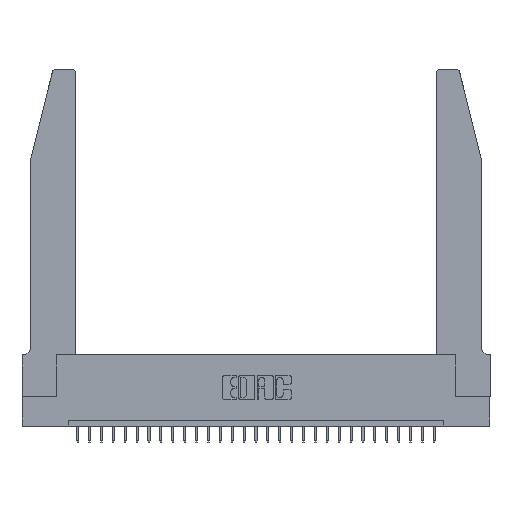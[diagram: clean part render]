
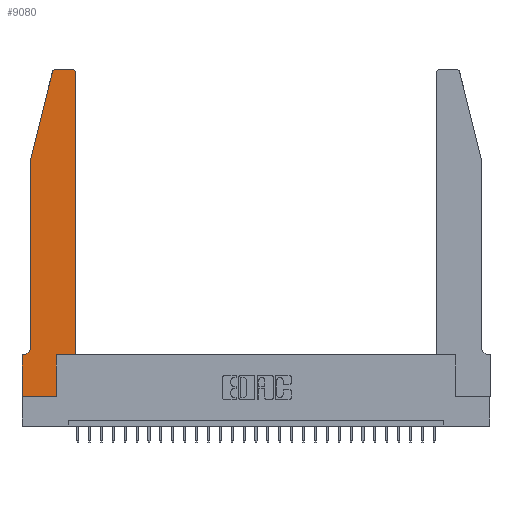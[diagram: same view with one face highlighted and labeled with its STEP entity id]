
A CAD part, top view. The second image highlights one B-rep face of the part: STEP entity #9080.
In plain terms, the highlighted planar face has unit normal (0, 0, 1).
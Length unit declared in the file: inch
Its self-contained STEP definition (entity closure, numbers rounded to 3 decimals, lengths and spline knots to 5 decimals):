
#590 = CARTESIAN_POINT ( 'NONE',  ( 0.0755, 2., 0.37 ) ) ;
#986 = VERTEX_POINT ( 'NONE', #4984 ) ;
#1604 = DIRECTION ( 'NONE',  ( 1., 0., 0. ) ) ;
#1984 = LINE ( 'NONE', #11432, #27392 ) ;
#2364 = EDGE_CURVE ( 'NONE', #3482, #9240, #22119, .T. ) ;
#2646 = ORIENTED_EDGE ( 'NONE', *, *, #24191, .T. ) ;
#3296 = DIRECTION ( 'NONE',  ( 0., 0., -1. ) ) ;
#3345 = AXIS2_PLACEMENT_3D ( 'NONE', #25358, #18606, #4831 ) ;
#3482 = VERTEX_POINT ( 'NONE', #4167 ) ;
#3673 = DIRECTION ( 'NONE',  ( -1., 0., 0. ) ) ;
#3963 = CARTESIAN_POINT ( 'NONE',  ( 0., 0.35, 0.37 ) ) ;
#4043 = CARTESIAN_POINT ( 'NONE',  ( 0.284, 2.75, 0.37 ) ) ;
#4167 = CARTESIAN_POINT ( 'NONE',  ( 0.4505, 0.35, 0.37 ) ) ;
#4831 = DIRECTION ( 'NONE',  ( 1., 0., 0. ) ) ;
#4951 = ORIENTED_EDGE ( 'NONE', *, *, #11667, .T. ) ;
#4984 = CARTESIAN_POINT ( 'NONE',  ( 0.0055, 0.35, 0.37 ) ) ;
#5324 = EDGE_LOOP ( 'NONE', ( #19766, #22884, #14265, #2646, #13859, #27532, #4951, #28599, #8783, #9372, #26543, #9269 ) ) ;
#6486 = VECTOR ( 'NONE', #26721, 39.37008 ) ;
#7499 = CARTESIAN_POINT ( 'NONE',  ( 0.4205, 2.72, 0.37 ) ) ;
#7570 = EDGE_CURVE ( 'NONE', #17487, #11560, #17320, .T. ) ;
#8108 = CIRCLE ( 'NONE', #3345, 0.03 ) ;
#8179 = VECTOR ( 'NONE', #23531, 39.37008 ) ;
#8783 = ORIENTED_EDGE ( 'NONE', *, *, #22785, .T. ) ;
#9080 = ADVANCED_FACE ( 'NONE', ( #18374 ), #13870, .T. ) ;
#9240 = VERTEX_POINT ( 'NONE', #28406 ) ;
#9269 = ORIENTED_EDGE ( 'NONE', *, *, #12693, .T. ) ;
#9277 = CARTESIAN_POINT ( 'NONE',  ( 0.0755, 0.35, 0.37 ) ) ;
#9372 = ORIENTED_EDGE ( 'NONE', *, *, #13191, .T. ) ;
#9401 = VERTEX_POINT ( 'NONE', #3963 ) ;
#9431 = DIRECTION ( 'NONE',  ( 0., -1., 0. ) ) ;
#9826 = CIRCLE ( 'NONE', #26076, 0.03 ) ;
#9972 = VECTOR ( 'NONE', #29241, 39.37008 ) ;
#10286 = VERTEX_POINT ( 'NONE', #27819 ) ;
#11387 = EDGE_CURVE ( 'NONE', #27579, #986, #11752, .T. ) ;
#11432 = CARTESIAN_POINT ( 'NONE',  ( 0.2865, 0.35, 0.37 ) ) ;
#11560 = VERTEX_POINT ( 'NONE', #4043 ) ;
#11566 = VECTOR ( 'NONE', #3673, 39.37008 ) ;
#11667 = EDGE_CURVE ( 'NONE', #9401, #10286, #15747, .T. ) ;
#11725 = DIRECTION ( 'NONE',  ( 0., 1., 0. ) ) ;
#11752 = CIRCLE ( 'NONE', #21312, 0.07 ) ;
#12062 = CARTESIAN_POINT ( 'NONE',  ( 0.25487, 2.72718, 0.37 ) ) ;
#12475 = VECTOR ( 'NONE', #27554, 39.37008 ) ;
#12693 = EDGE_CURVE ( 'NONE', #9240, #17487, #9826, .T. ) ;
#12758 = VERTEX_POINT ( 'NONE', #21304 ) ;
#13191 = EDGE_CURVE ( 'NONE', #25428, #3482, #19703, .T. ) ;
#13729 = DIRECTION ( 'NONE',  ( 0., 0., 1. ) ) ;
#13859 = ORIENTED_EDGE ( 'NONE', *, *, #11387, .T. ) ;
#13870 = PLANE ( 'NONE',  #27821 ) ;
#13918 = VECTOR ( 'NONE', #1604, 39.37008 ) ;
#14265 = ORIENTED_EDGE ( 'NONE', *, *, #21430, .T. ) ;
#14365 = VERTEX_POINT ( 'NONE', #16455 ) ;
#14915 = CARTESIAN_POINT ( 'NONE',  ( 0.2605, 2.75, 0.37 ) ) ;
#15747 = LINE ( 'NONE', #25028, #26099 ) ;
#16148 = DIRECTION ( 'NONE',  ( 1., 0., 0. ) ) ;
#16455 = CARTESIAN_POINT ( 'NONE',  ( 0.0755, 2., 0.37 ) ) ;
#17320 = LINE ( 'NONE', #14915, #11566 ) ;
#17487 = VERTEX_POINT ( 'NONE', #24387 ) ;
#17632 = DIRECTION ( 'NONE',  ( 0., 1., 0. ) ) ;
#18374 = FACE_OUTER_BOUND ( 'NONE', #5324, .T. ) ;
#18606 = DIRECTION ( 'NONE',  ( 0., 0., 1. ) ) ;
#18880 = CARTESIAN_POINT ( 'NONE',  ( 0.0755, 0.42, 0.37 ) ) ;
#18900 = DIRECTION ( 'NONE',  ( -1., 0., 0. ) ) ;
#19360 = DIRECTION ( 'NONE',  ( 1., 0., 0. ) ) ;
#19433 = CARTESIAN_POINT ( 'NONE',  ( 0.2865, 0.35, 0.37 ) ) ;
#19657 = CARTESIAN_POINT ( 'NONE',  ( 0.0755, 2., 0.37 ) ) ;
#19703 = LINE ( 'NONE', #26266, #6486 ) ;
#19766 = ORIENTED_EDGE ( 'NONE', *, *, #7570, .T. ) ;
#19945 = EDGE_CURVE ( 'NONE', #11560, #23653, #8108, .T. ) ;
#20494 = CARTESIAN_POINT ( 'NONE',  ( 0., 0.35, 0.37 ) ) ;
#21304 = CARTESIAN_POINT ( 'NONE',  ( 0.2865, 0., 0.37 ) ) ;
#21312 = AXIS2_PLACEMENT_3D ( 'NONE', #23970, #3296, #18900 ) ;
#21430 = EDGE_CURVE ( 'NONE', #23653, #14365, #25761, .T. ) ;
#22119 = LINE ( 'NONE', #24361, #25540 ) ;
#22139 = LINE ( 'NONE', #24077, #13918 ) ;
#22785 = EDGE_CURVE ( 'NONE', #12758, #25428, #1984, .T. ) ;
#22884 = ORIENTED_EDGE ( 'NONE', *, *, #19945, .T. ) ;
#22906 = LINE ( 'NONE', #9277, #12475 ) ;
#23531 = DIRECTION ( 'NONE',  ( -0.239, -0.971, 0. ) ) ;
#23653 = VERTEX_POINT ( 'NONE', #12062 ) ;
#23970 = CARTESIAN_POINT ( 'NONE',  ( 0.0055, 0.42, 0.37 ) ) ;
#24077 = CARTESIAN_POINT ( 'NONE',  ( 0., 0., 0.37 ) ) ;
#24191 = EDGE_CURVE ( 'NONE', #14365, #27579, #28792, .T. ) ;
#24361 = CARTESIAN_POINT ( 'NONE',  ( 0.4505, 0.35, 0.37 ) ) ;
#24387 = CARTESIAN_POINT ( 'NONE',  ( 0.4205, 2.75, 0.37 ) ) ;
#25028 = CARTESIAN_POINT ( 'NONE',  ( 0., 0., 0.37 ) ) ;
#25358 = CARTESIAN_POINT ( 'NONE',  ( 0.284, 2.72, 0.37 ) ) ;
#25428 = VERTEX_POINT ( 'NONE', #19433 ) ;
#25540 = VECTOR ( 'NONE', #17632, 39.37008 ) ;
#25761 = LINE ( 'NONE', #590, #8179 ) ;
#26076 = AXIS2_PLACEMENT_3D ( 'NONE', #7499, #26367, #19360 ) ;
#26099 = VECTOR ( 'NONE', #9431, 39.37008 ) ;
#26266 = CARTESIAN_POINT ( 'NONE',  ( 0.4505, 0.35, 0.37 ) ) ;
#26367 = DIRECTION ( 'NONE',  ( 0., 0., 1. ) ) ;
#26543 = ORIENTED_EDGE ( 'NONE', *, *, #2364, .T. ) ;
#26721 = DIRECTION ( 'NONE',  ( 1., 0., 0. ) ) ;
#27392 = VECTOR ( 'NONE', #11725, 39.37008 ) ;
#27532 = ORIENTED_EDGE ( 'NONE', *, *, #29073, .T. ) ;
#27554 = DIRECTION ( 'NONE',  ( -1., 0., 0. ) ) ;
#27579 = VERTEX_POINT ( 'NONE', #18880 ) ;
#27819 = CARTESIAN_POINT ( 'NONE',  ( 0., 0., 0.37 ) ) ;
#27821 = AXIS2_PLACEMENT_3D ( 'NONE', #20494, #13729, #16148 ) ;
#28406 = CARTESIAN_POINT ( 'NONE',  ( 0.4505, 2.72, 0.37 ) ) ;
#28599 = ORIENTED_EDGE ( 'NONE', *, *, #29426, .T. ) ;
#28792 = LINE ( 'NONE', #19657, #9972 ) ;
#29073 = EDGE_CURVE ( 'NONE', #986, #9401, #22906, .T. ) ;
#29241 = DIRECTION ( 'NONE',  ( 0., -1., 0. ) ) ;
#29426 = EDGE_CURVE ( 'NONE', #10286, #12758, #22139, .T. ) ;
